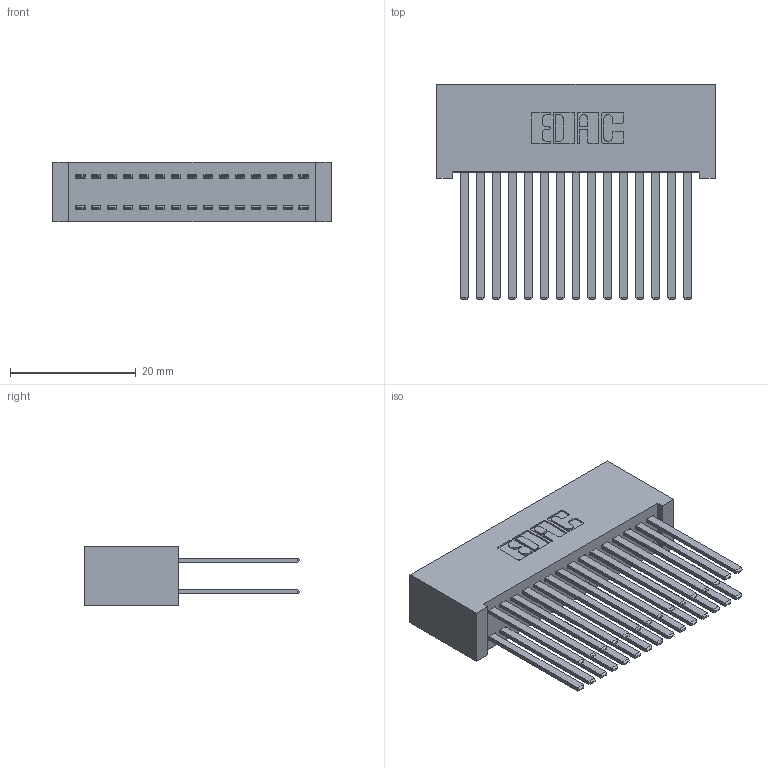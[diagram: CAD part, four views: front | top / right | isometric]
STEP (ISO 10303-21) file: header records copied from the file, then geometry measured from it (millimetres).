
FILE_DESCRIPTION (( 'STEP AP203' ), '1' );
FILE_NAME ('392-030-544-201.STEP', '2018-08-15T22:42:12', ( '' ), ( '' ), 'SwSTEP 2.0', 'SolidWorks 2016', '' );
FILE_SCHEMA (( 'CONFIG_CONTROL_DESIGN' ));
Length unit declared in the file: inch
Products named in the file (3): 342 Part_Lugless; 392-030-544-201; 345-292-001_345-293-144
Assembly tree (31 placements, depth 2):
  392-030-544-201
    342 Part_Lugless
    345-292-001_345-293-144  x30
Bounding box: 44.35 x 34.3 x 9.4 mm (x, y, z)
Volume: 4717 mm3; surface area: 8623.6 mm2
Topology: 31 solids, 31 shells, 1482 faces, 4385 edges, 2882 vertices
Faces by surface type: plane 1022, cylinder 460
Entity records: 12549 total; most frequent: CARTESIAN_POINT 2106, ORIENTED_EDGE 2042, DIRECTION 1837, EDGE_CURVE 1021, LINE 905, VECTOR 905, VERTEX_POINT 678, AXIS2_PLACEMENT_3D 466
